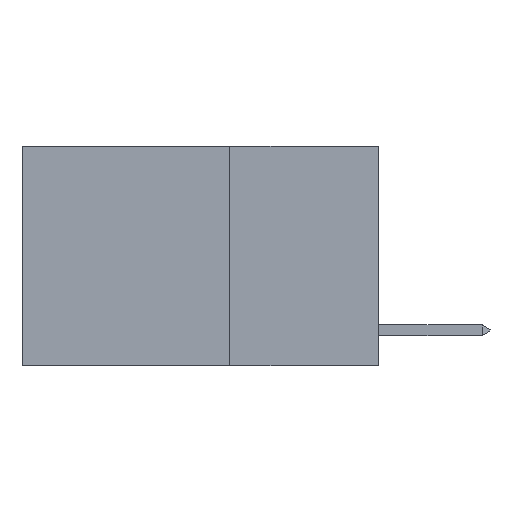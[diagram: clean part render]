
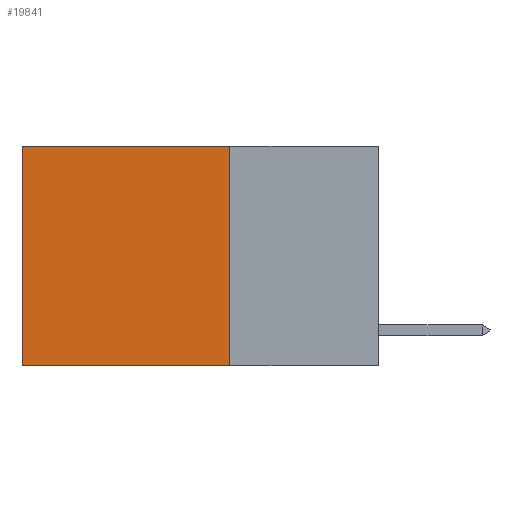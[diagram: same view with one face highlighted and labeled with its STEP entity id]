
A CAD part, left-side view. The second image highlights one B-rep face of the part: STEP entity #19841.
In plain terms, the highlighted planar face has unit normal (-1, 0, 0).
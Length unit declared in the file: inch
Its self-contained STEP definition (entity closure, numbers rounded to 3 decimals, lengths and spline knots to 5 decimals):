
#135 = CARTESIAN_POINT ( 'NONE',  ( 0.2625, 0.25, 0. ) ) ;
#733 = EDGE_CURVE ( 'NONE', #2867, #10297, #3707, .T. ) ;
#2125 = VECTOR ( 'NONE', #2329, 39.37008 ) ;
#2329 = DIRECTION ( 'NONE',  ( 0., 1., 0. ) ) ;
#2589 = EDGE_CURVE ( 'NONE', #10297, #14728, #14738, .T. ) ;
#2867 = VERTEX_POINT ( 'NONE', #135 ) ;
#2929 = ORIENTED_EDGE ( 'NONE', *, *, #2589, .F. ) ;
#3296 = LINE ( 'NONE', #5316, #7028 ) ;
#3707 = LINE ( 'NONE', #7126, #11658 ) ;
#5275 = EDGE_CURVE ( 'NONE', #6835, #14728, #3296, .T. ) ;
#5316 = CARTESIAN_POINT ( 'NONE',  ( 0.2625, 0.6, 0. ) ) ;
#5548 = ORIENTED_EDGE ( 'NONE', *, *, #8592, .T. ) ;
#6834 = DIRECTION ( 'NONE',  ( 1., 0., 0. ) ) ;
#6835 = VERTEX_POINT ( 'NONE', #18620 ) ;
#6925 = DIRECTION ( 'NONE',  ( 0., 0., -1. ) ) ;
#7028 = VECTOR ( 'NONE', #6925, 39.37008 ) ;
#7126 = CARTESIAN_POINT ( 'NONE',  ( 0.2625, 0.25, 0. ) ) ;
#7342 = AXIS2_PLACEMENT_3D ( 'NONE', #14663, #6834, #17778 ) ;
#8592 = EDGE_CURVE ( 'NONE', #2867, #6835, #14565, .T. ) ;
#9170 = FACE_OUTER_BOUND ( 'NONE', #13282, .T. ) ;
#9570 = DIRECTION ( 'NONE',  ( 0., 0., -1. ) ) ;
#10297 = VERTEX_POINT ( 'NONE', #19610 ) ;
#10438 = VECTOR ( 'NONE', #16580, 39.37008 ) ;
#11658 = VECTOR ( 'NONE', #9570, 39.37008 ) ;
#12661 = ORIENTED_EDGE ( 'NONE', *, *, #5275, .T. ) ;
#13123 = ORIENTED_EDGE ( 'NONE', *, *, #733, .F. ) ;
#13282 = EDGE_LOOP ( 'NONE', ( #12661, #2929, #13123, #5548 ) ) ;
#14565 = LINE ( 'NONE', #18191, #10438 ) ;
#14663 = CARTESIAN_POINT ( 'NONE',  ( 0.2625, 0.25, 0. ) ) ;
#14728 = VERTEX_POINT ( 'NONE', #16983 ) ;
#14738 = LINE ( 'NONE', #19554, #2125 ) ;
#16580 = DIRECTION ( 'NONE',  ( 0., 1., 0. ) ) ;
#16983 = CARTESIAN_POINT ( 'NONE',  ( 0.2625, 0.6, -0.37 ) ) ;
#17708 = PLANE ( 'NONE',  #7342 ) ;
#17778 = DIRECTION ( 'NONE',  ( 0., 0., -1. ) ) ;
#18191 = CARTESIAN_POINT ( 'NONE',  ( 0.2625, 0.25, 0. ) ) ;
#18620 = CARTESIAN_POINT ( 'NONE',  ( 0.2625, 0.6, 0. ) ) ;
#19554 = CARTESIAN_POINT ( 'NONE',  ( 0.2625, 0.25, -0.37 ) ) ;
#19610 = CARTESIAN_POINT ( 'NONE',  ( 0.2625, 0.25, -0.37 ) ) ;
#19841 = ADVANCED_FACE ( 'NONE', ( #9170 ), #17708, .F. ) ;
